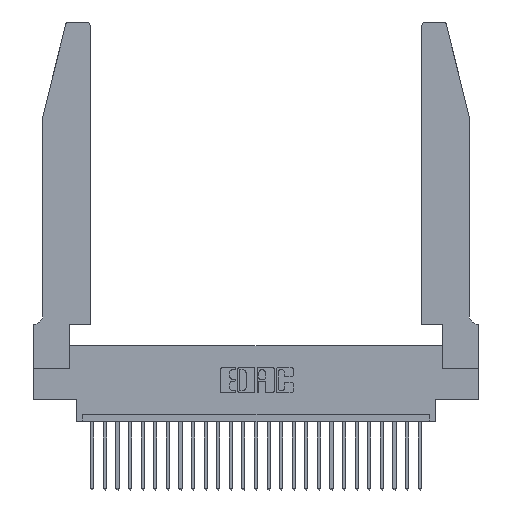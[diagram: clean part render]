
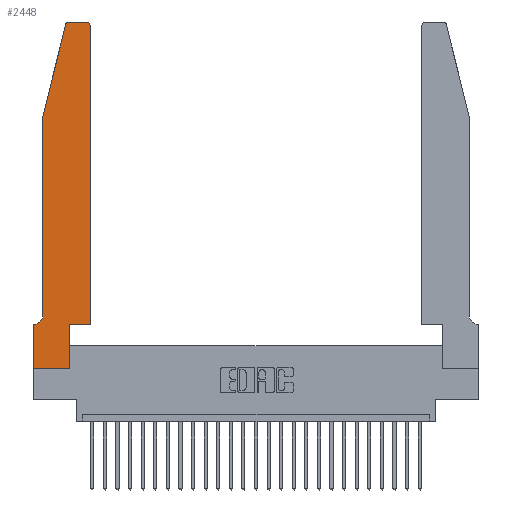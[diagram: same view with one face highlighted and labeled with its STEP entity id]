
A CAD part, top view. The second image highlights one B-rep face of the part: STEP entity #2448.
In plain terms, the highlighted planar face has unit normal (0, 0, 1).
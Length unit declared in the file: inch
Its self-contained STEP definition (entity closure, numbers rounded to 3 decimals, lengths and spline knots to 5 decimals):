
#307 = LINE ( 'NONE', #7585, #22022 ) ;
#1456 = CARTESIAN_POINT ( 'NONE',  ( 0.4505, 0.35, 0.37 ) ) ;
#1463 = DIRECTION ( 'NONE',  ( 0., 0., -1. ) ) ;
#1662 = DIRECTION ( 'NONE',  ( 0., -1., 0. ) ) ;
#1705 = ORIENTED_EDGE ( 'NONE', *, *, #4433, .T. ) ;
#1833 = ORIENTED_EDGE ( 'NONE', *, *, #20567, .T. ) ;
#2318 = VECTOR ( 'NONE', #11578, 39.37008 ) ;
#2448 = ADVANCED_FACE ( 'NONE', ( #10713 ), #12112, .T. ) ;
#2711 = ORIENTED_EDGE ( 'NONE', *, *, #6495, .T. ) ;
#3415 = DIRECTION ( 'NONE',  ( -0.239, -0.971, 0. ) ) ;
#3654 = ORIENTED_EDGE ( 'NONE', *, *, #3769, .T. ) ;
#3769 = EDGE_CURVE ( 'NONE', #21100, #24241, #11647, .T. ) ;
#4433 = EDGE_CURVE ( 'NONE', #18867, #14497, #24755, .T. ) ;
#4506 = ORIENTED_EDGE ( 'NONE', *, *, #4930, .T. ) ;
#4930 = EDGE_CURVE ( 'NONE', #14497, #17096, #26669, .T. ) ;
#4947 = VECTOR ( 'NONE', #13210, 39.37008 ) ;
#5062 = CARTESIAN_POINT ( 'NONE',  ( 0.4205, 2.72, 0.37 ) ) ;
#5110 = VERTEX_POINT ( 'NONE', #22706 ) ;
#5134 = VECTOR ( 'NONE', #3415, 39.37008 ) ;
#5276 = CARTESIAN_POINT ( 'NONE',  ( 0.0755, 2., 0.37 ) ) ;
#5352 = CARTESIAN_POINT ( 'NONE',  ( 0.284, 2.72, 0.37 ) ) ;
#5936 = ORIENTED_EDGE ( 'NONE', *, *, #14261, .T. ) ;
#6463 = CARTESIAN_POINT ( 'NONE',  ( 0.4205, 2.75, 0.37 ) ) ;
#6495 = EDGE_CURVE ( 'NONE', #5110, #22795, #13440, .T. ) ;
#6641 = CARTESIAN_POINT ( 'NONE',  ( 0., 0.35, 0.37 ) ) ;
#6736 = CARTESIAN_POINT ( 'NONE',  ( 0.2865, 0., 0.37 ) ) ;
#6921 = ORIENTED_EDGE ( 'NONE', *, *, #18887, .T. ) ;
#7206 = DIRECTION ( 'NONE',  ( -1., 0., 0. ) ) ;
#7322 = VECTOR ( 'NONE', #23913, 39.37008 ) ;
#7585 = CARTESIAN_POINT ( 'NONE',  ( 0.4505, 0.35, 0.37 ) ) ;
#7682 = EDGE_CURVE ( 'NONE', #10558, #21100, #13824, .T. ) ;
#8038 = DIRECTION ( 'NONE',  ( 0., 0., 1. ) ) ;
#8123 = LINE ( 'NONE', #9517, #5134 ) ;
#8169 = CIRCLE ( 'NONE', #13358, 0.03 ) ;
#9106 = VERTEX_POINT ( 'NONE', #17931 ) ;
#9169 = CARTESIAN_POINT ( 'NONE',  ( 0.4505, 2.72, 0.37 ) ) ;
#9315 = CARTESIAN_POINT ( 'NONE',  ( 0., 0., 0.37 ) ) ;
#9423 = DIRECTION ( 'NONE',  ( 0., 0., 1. ) ) ;
#9517 = CARTESIAN_POINT ( 'NONE',  ( 0.0755, 2., 0.37 ) ) ;
#9593 = DIRECTION ( 'NONE',  ( -1., 0., 0. ) ) ;
#9635 = LINE ( 'NONE', #13073, #7322 ) ;
#9916 = CARTESIAN_POINT ( 'NONE',  ( 0.2865, 0.35, 0.37 ) ) ;
#10296 = CARTESIAN_POINT ( 'NONE',  ( 0.2865, 0.35, 0.37 ) ) ;
#10558 = VERTEX_POINT ( 'NONE', #17944 ) ;
#10588 = LINE ( 'NONE', #15432, #4947 ) ;
#10713 = FACE_OUTER_BOUND ( 'NONE', #21813, .T. ) ;
#10879 = VECTOR ( 'NONE', #7206, 39.37008 ) ;
#11149 = ORIENTED_EDGE ( 'NONE', *, *, #14919, .T. ) ;
#11533 = LINE ( 'NONE', #5276, #2318 ) ;
#11578 = DIRECTION ( 'NONE',  ( 0., -1., 0. ) ) ;
#11647 = LINE ( 'NONE', #9315, #25787 ) ;
#12112 = PLANE ( 'NONE',  #24941 ) ;
#13073 = CARTESIAN_POINT ( 'NONE',  ( 0.2605, 2.75, 0.37 ) ) ;
#13210 = DIRECTION ( 'NONE',  ( 1., 0., 0. ) ) ;
#13347 = EDGE_CURVE ( 'NONE', #14659, #5110, #9635, .T. ) ;
#13358 = AXIS2_PLACEMENT_3D ( 'NONE', #5062, #9423, #22271 ) ;
#13371 = CIRCLE ( 'NONE', #14248, 0.07 ) ;
#13440 = CIRCLE ( 'NONE', #19552, 0.03 ) ;
#13484 = CARTESIAN_POINT ( 'NONE',  ( 0.0755, 0.35, 0.37 ) ) ;
#13824 = LINE ( 'NONE', #13484, #10879 ) ;
#14025 = ORIENTED_EDGE ( 'NONE', *, *, #16124, .T. ) ;
#14051 = CARTESIAN_POINT ( 'NONE',  ( 0.0755, 0.42, 0.37 ) ) ;
#14248 = AXIS2_PLACEMENT_3D ( 'NONE', #24385, #1463, #9593 ) ;
#14261 = EDGE_CURVE ( 'NONE', #26000, #14659, #8169, .T. ) ;
#14275 = DIRECTION ( 'NONE',  ( 1., 0., 0. ) ) ;
#14402 = VERTEX_POINT ( 'NONE', #14051 ) ;
#14497 = VERTEX_POINT ( 'NONE', #9916 ) ;
#14659 = VERTEX_POINT ( 'NONE', #6463 ) ;
#14919 = EDGE_CURVE ( 'NONE', #22795, #9106, #8123, .T. ) ;
#15157 = CARTESIAN_POINT ( 'NONE',  ( 0.25487, 2.72718, 0.37 ) ) ;
#15368 = DIRECTION ( 'NONE',  ( 0., 1., 0. ) ) ;
#15432 = CARTESIAN_POINT ( 'NONE',  ( 0., 0., 0.37 ) ) ;
#15438 = CARTESIAN_POINT ( 'NONE',  ( 0., 0., 0.37 ) ) ;
#15534 = VECTOR ( 'NONE', #14275, 39.37008 ) ;
#15576 = VECTOR ( 'NONE', #15704, 39.37008 ) ;
#15704 = DIRECTION ( 'NONE',  ( 0., 1., 0. ) ) ;
#16124 = EDGE_CURVE ( 'NONE', #14402, #10558, #13371, .T. ) ;
#17033 = ORIENTED_EDGE ( 'NONE', *, *, #20166, .T. ) ;
#17096 = VERTEX_POINT ( 'NONE', #1456 ) ;
#17341 = ORIENTED_EDGE ( 'NONE', *, *, #13347, .T. ) ;
#17931 = CARTESIAN_POINT ( 'NONE',  ( 0.0755, 2., 0.37 ) ) ;
#17944 = CARTESIAN_POINT ( 'NONE',  ( 0.0055, 0.35, 0.37 ) ) ;
#18333 = ORIENTED_EDGE ( 'NONE', *, *, #7682, .T. ) ;
#18867 = VERTEX_POINT ( 'NONE', #6736 ) ;
#18887 = EDGE_CURVE ( 'NONE', #24241, #18867, #10588, .T. ) ;
#19552 = AXIS2_PLACEMENT_3D ( 'NONE', #5352, #26172, #22598 ) ;
#20166 = EDGE_CURVE ( 'NONE', #9106, #14402, #11533, .T. ) ;
#20255 = DIRECTION ( 'NONE',  ( 1., 0., 0. ) ) ;
#20567 = EDGE_CURVE ( 'NONE', #17096, #26000, #307, .T. ) ;
#21100 = VERTEX_POINT ( 'NONE', #6641 ) ;
#21813 = EDGE_LOOP ( 'NONE', ( #17341, #2711, #11149, #17033, #14025, #18333, #3654, #6921, #1705, #4506, #1833, #5936 ) ) ;
#22022 = VECTOR ( 'NONE', #15368, 39.37008 ) ;
#22271 = DIRECTION ( 'NONE',  ( 1., 0., 0. ) ) ;
#22598 = DIRECTION ( 'NONE',  ( 1., 0., 0. ) ) ;
#22706 = CARTESIAN_POINT ( 'NONE',  ( 0.284, 2.75, 0.37 ) ) ;
#22795 = VERTEX_POINT ( 'NONE', #15157 ) ;
#22826 = CARTESIAN_POINT ( 'NONE',  ( 0.4505, 0.35, 0.37 ) ) ;
#23913 = DIRECTION ( 'NONE',  ( -1., 0., 0. ) ) ;
#24241 = VERTEX_POINT ( 'NONE', #15438 ) ;
#24385 = CARTESIAN_POINT ( 'NONE',  ( 0.0055, 0.42, 0.37 ) ) ;
#24755 = LINE ( 'NONE', #10296, #15576 ) ;
#24772 = CARTESIAN_POINT ( 'NONE',  ( 0., 0.35, 0.37 ) ) ;
#24941 = AXIS2_PLACEMENT_3D ( 'NONE', #24772, #8038, #20255 ) ;
#25787 = VECTOR ( 'NONE', #1662, 39.37008 ) ;
#26000 = VERTEX_POINT ( 'NONE', #9169 ) ;
#26172 = DIRECTION ( 'NONE',  ( 0., 0., 1. ) ) ;
#26669 = LINE ( 'NONE', #22826, #15534 ) ;
